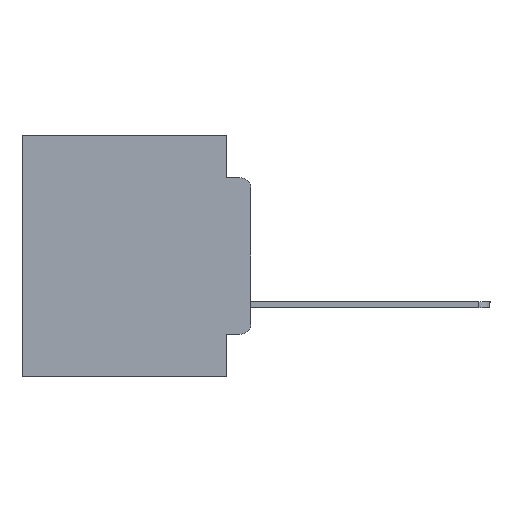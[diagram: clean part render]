
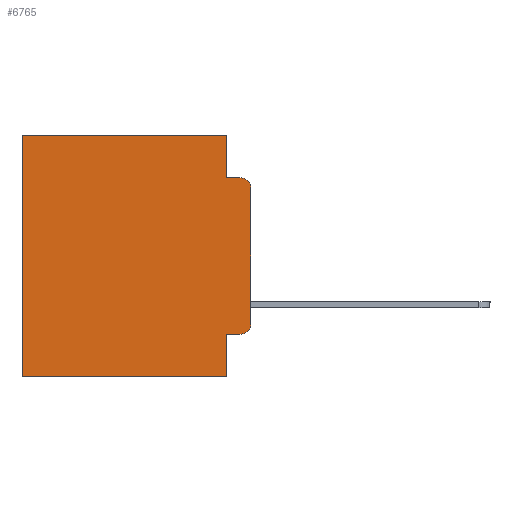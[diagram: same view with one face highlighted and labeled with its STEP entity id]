
A CAD part, left-side view. The second image highlights one B-rep face of the part: STEP entity #6765.
In plain terms, the highlighted planar face has unit normal (-1, 0, 0).
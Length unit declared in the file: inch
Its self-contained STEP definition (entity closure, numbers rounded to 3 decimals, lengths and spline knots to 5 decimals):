
#297 = CARTESIAN_POINT ( 'NONE',  ( 0.298, 0.051, -0.4115 ) ) ;
#1109 = LINE ( 'NONE', #21914, #19480 ) ;
#1269 = CARTESIAN_POINT ( 'NONE',  ( 0.298, 0.051, -0.4115 ) ) ;
#1518 = VERTEX_POINT ( 'NONE', #18511 ) ;
#2467 = CARTESIAN_POINT ( 'NONE',  ( 0.298, 0.02, -0.4115 ) ) ;
#2674 = VECTOR ( 'NONE', #25533, 39.37008 ) ;
#3175 = CARTESIAN_POINT ( 'NONE',  ( 0.298, 0.051, -0.0885 ) ) ;
#3180 = EDGE_CURVE ( 'NONE', #17108, #4362, #14151, .T. ) ;
#4362 = VERTEX_POINT ( 'NONE', #11451 ) ;
#4875 = CARTESIAN_POINT ( 'NONE',  ( 0.298, 0.051, 0. ) ) ;
#5315 = EDGE_CURVE ( 'NONE', #18287, #21520, #10709, .T. ) ;
#5333 = VECTOR ( 'NONE', #5967, 39.37008 ) ;
#5613 = VECTOR ( 'NONE', #24016, 39.37008 ) ;
#5967 = DIRECTION ( 'NONE',  ( 0., 1., 0. ) ) ;
#6403 = DIRECTION ( 'NONE',  ( 0., -1., 0. ) ) ;
#6436 = CARTESIAN_POINT ( 'NONE',  ( 0.298, 0.051, -0.0885 ) ) ;
#6765 = ADVANCED_FACE ( 'NONE', ( #24326 ), #16140, .F. ) ;
#6919 = CIRCLE ( 'NONE', #9951, 0.02 ) ;
#7163 = AXIS2_PLACEMENT_3D ( 'NONE', #7729, #20772, #22290 ) ;
#7314 = CARTESIAN_POINT ( 'NONE',  ( 0.298, 0., 0. ) ) ;
#7658 = ORIENTED_EDGE ( 'NONE', *, *, #16567, .T. ) ;
#7729 = CARTESIAN_POINT ( 'NONE',  ( 0.298, 0.02, -0.3915 ) ) ;
#7757 = VECTOR ( 'NONE', #6403, 39.37008 ) ;
#8564 = LINE ( 'NONE', #20931, #23428 ) ;
#8944 = VERTEX_POINT ( 'NONE', #1269 ) ;
#9162 = EDGE_CURVE ( 'NONE', #13367, #16793, #1109, .T. ) ;
#9587 = VECTOR ( 'NONE', #13477, 39.37008 ) ;
#9812 = CARTESIAN_POINT ( 'NONE',  ( 0.298, 0.051, 0. ) ) ;
#9951 = AXIS2_PLACEMENT_3D ( 'NONE', #23889, #17348, #19659 ) ;
#10359 = LINE ( 'NONE', #297, #7757 ) ;
#10709 = LINE ( 'NONE', #4875, #15017 ) ;
#10754 = EDGE_CURVE ( 'NONE', #24452, #16793, #14129, .T. ) ;
#11152 = LINE ( 'NONE', #19441, #9587 ) ;
#11451 = CARTESIAN_POINT ( 'NONE',  ( 0.298, 0.473, -0.5 ) ) ;
#12362 = ORIENTED_EDGE ( 'NONE', *, *, #3180, .F. ) ;
#12609 = ORIENTED_EDGE ( 'NONE', *, *, #23611, .F. ) ;
#12787 = EDGE_CURVE ( 'NONE', #13367, #17197, #6919, .T. ) ;
#13138 = CARTESIAN_POINT ( 'NONE',  ( 0.298, 0.473, 0. ) ) ;
#13250 = LINE ( 'NONE', #3175, #5613 ) ;
#13319 = AXIS2_PLACEMENT_3D ( 'NONE', #7314, #20346, #15625 ) ;
#13367 = VERTEX_POINT ( 'NONE', #14225 ) ;
#13477 = DIRECTION ( 'NONE',  ( 0., 1., 0. ) ) ;
#14129 = CIRCLE ( 'NONE', #7163, 0.02 ) ;
#14151 = LINE ( 'NONE', #18620, #5333 ) ;
#14225 = CARTESIAN_POINT ( 'NONE',  ( 0.298, 0., -0.1085 ) ) ;
#14266 = ORIENTED_EDGE ( 'NONE', *, *, #24200, .F. ) ;
#14957 = ORIENTED_EDGE ( 'NONE', *, *, #9162, .F. ) ;
#15017 = VECTOR ( 'NONE', #23525, 39.37008 ) ;
#15625 = DIRECTION ( 'NONE',  ( 0., 0., -1. ) ) ;
#15767 = EDGE_CURVE ( 'NONE', #18287, #1518, #11152, .T. ) ;
#15919 = ORIENTED_EDGE ( 'NONE', *, *, #10754, .T. ) ;
#16140 = PLANE ( 'NONE',  #13319 ) ;
#16567 = EDGE_CURVE ( 'NONE', #1518, #4362, #19378, .T. ) ;
#16591 = DIRECTION ( 'NONE',  ( 0., 0., -1. ) ) ;
#16793 = VERTEX_POINT ( 'NONE', #18827 ) ;
#17108 = VERTEX_POINT ( 'NONE', #20016 ) ;
#17197 = VERTEX_POINT ( 'NONE', #22323 ) ;
#17348 = DIRECTION ( 'NONE',  ( -1., 0., 0. ) ) ;
#17835 = DIRECTION ( 'NONE',  ( 0., 0., -1. ) ) ;
#18287 = VERTEX_POINT ( 'NONE', #9812 ) ;
#18405 = ORIENTED_EDGE ( 'NONE', *, *, #5315, .F. ) ;
#18455 = ORIENTED_EDGE ( 'NONE', *, *, #23215, .T. ) ;
#18511 = CARTESIAN_POINT ( 'NONE',  ( 0.298, 0.473, 0. ) ) ;
#18620 = CARTESIAN_POINT ( 'NONE',  ( 0.298, 0., -0.5 ) ) ;
#18827 = CARTESIAN_POINT ( 'NONE',  ( 0.298, 0., -0.3915 ) ) ;
#19378 = LINE ( 'NONE', #13138, #2674 ) ;
#19441 = CARTESIAN_POINT ( 'NONE',  ( 0.298, 0., 0. ) ) ;
#19480 = VECTOR ( 'NONE', #17835, 39.37008 ) ;
#19659 = DIRECTION ( 'NONE',  ( 0., 0., -1. ) ) ;
#20016 = CARTESIAN_POINT ( 'NONE',  ( 0.298, 0.051, -0.5 ) ) ;
#20346 = DIRECTION ( 'NONE',  ( 1., 0., 0. ) ) ;
#20772 = DIRECTION ( 'NONE',  ( -1., 0., 0. ) ) ;
#20931 = CARTESIAN_POINT ( 'NONE',  ( 0.298, 0.051, 0. ) ) ;
#21520 = VERTEX_POINT ( 'NONE', #6436 ) ;
#21914 = CARTESIAN_POINT ( 'NONE',  ( 0.298, 0., 0. ) ) ;
#22275 = ORIENTED_EDGE ( 'NONE', *, *, #15767, .T. ) ;
#22290 = DIRECTION ( 'NONE',  ( 0., 0., -1. ) ) ;
#22323 = CARTESIAN_POINT ( 'NONE',  ( 0.298, 0.02, -0.0885 ) ) ;
#23215 = EDGE_CURVE ( 'NONE', #8944, #24452, #10359, .T. ) ;
#23428 = VECTOR ( 'NONE', #16591, 39.37008 ) ;
#23525 = DIRECTION ( 'NONE',  ( 0., 0., -1. ) ) ;
#23611 = EDGE_CURVE ( 'NONE', #8944, #17108, #8564, .T. ) ;
#23889 = CARTESIAN_POINT ( 'NONE',  ( 0.298, 0.02, -0.1085 ) ) ;
#24016 = DIRECTION ( 'NONE',  ( 0., -1., 0. ) ) ;
#24021 = EDGE_LOOP ( 'NONE', ( #14957, #24753, #14266, #18405, #22275, #7658, #12362, #12609, #18455, #15919 ) ) ;
#24200 = EDGE_CURVE ( 'NONE', #21520, #17197, #13250, .T. ) ;
#24326 = FACE_OUTER_BOUND ( 'NONE', #24021, .T. ) ;
#24452 = VERTEX_POINT ( 'NONE', #2467 ) ;
#24753 = ORIENTED_EDGE ( 'NONE', *, *, #12787, .T. ) ;
#25533 = DIRECTION ( 'NONE',  ( 0., 0., -1. ) ) ;
